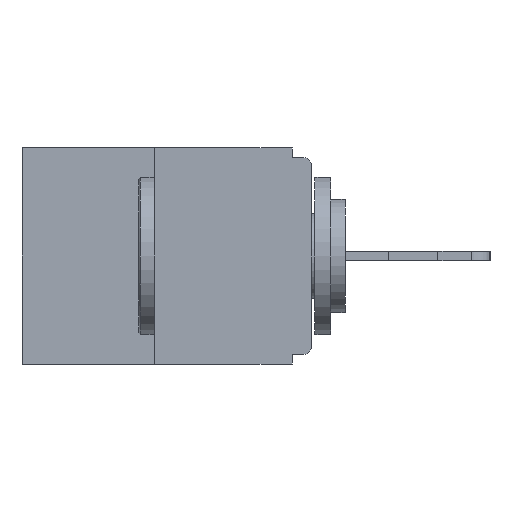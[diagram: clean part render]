
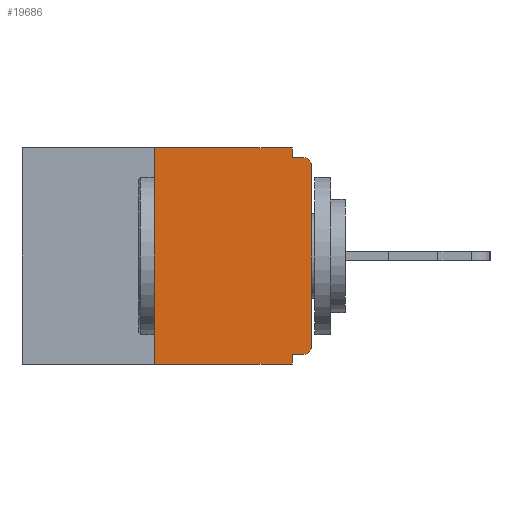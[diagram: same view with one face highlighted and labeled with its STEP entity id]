
A CAD part, left-side view. The second image highlights one B-rep face of the part: STEP entity #19686.
In plain terms, the highlighted planar face has unit normal (-1, 0, 0).
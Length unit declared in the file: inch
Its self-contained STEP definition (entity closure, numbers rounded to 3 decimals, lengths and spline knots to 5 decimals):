
#166 = EDGE_CURVE ( 'NONE', #26643, #11274, #13136, .T. ) ;
#440 = AXIS2_PLACEMENT_3D ( 'NONE', #13246, #17662, #4589 ) ;
#574 = VERTEX_POINT ( 'NONE', #23332 ) ;
#845 = VECTOR ( 'NONE', #21082, 39.37008 ) ;
#1140 = ORIENTED_EDGE ( 'NONE', *, *, #15263, .F. ) ;
#2110 = DIRECTION ( 'NONE',  ( 0., 0., 1. ) ) ;
#2304 = CARTESIAN_POINT ( 'NONE',  ( 0., 0.015, -0.328 ) ) ;
#2438 = AXIS2_PLACEMENT_3D ( 'NONE', #19368, #6268, #21599 ) ;
#2538 = EDGE_CURVE ( 'NONE', #574, #8036, #25478, .T. ) ;
#3503 = LINE ( 'NONE', #9807, #14394 ) ;
#3701 = EDGE_CURVE ( 'NONE', #25444, #11274, #28105, .T. ) ;
#4238 = CARTESIAN_POINT ( 'NONE',  ( 0., 0.25, 0. ) ) ;
#4418 = LINE ( 'NONE', #28301, #27008 ) ;
#4589 = DIRECTION ( 'NONE',  ( 0., 0., -1. ) ) ;
#4833 = CARTESIAN_POINT ( 'NONE',  ( 0., 0., -0.313 ) ) ;
#4880 = EDGE_CURVE ( 'NONE', #6630, #25444, #8194, .T. ) ;
#5594 = CARTESIAN_POINT ( 'NONE',  ( 0., 0.46, 0. ) ) ;
#5620 = ORIENTED_EDGE ( 'NONE', *, *, #4880, .F. ) ;
#5978 = VECTOR ( 'NONE', #16418, 39.37008 ) ;
#6268 = DIRECTION ( 'NONE',  ( -1., 0., 0. ) ) ;
#6456 = DIRECTION ( 'NONE',  ( -1., 0., 0. ) ) ;
#6630 = VERTEX_POINT ( 'NONE', #2304 ) ;
#6703 = PLANE ( 'NONE',  #440 ) ;
#7057 = CARTESIAN_POINT ( 'NONE',  ( 0., 0., -0.328 ) ) ;
#7600 = CARTESIAN_POINT ( 'NONE',  ( 0., 0.015, -0.015 ) ) ;
#7668 = ORIENTED_EDGE ( 'NONE', *, *, #166, .T. ) ;
#7722 = EDGE_CURVE ( 'NONE', #6630, #25954, #27837, .T. ) ;
#8036 = VERTEX_POINT ( 'NONE', #7600 ) ;
#8194 = LINE ( 'NONE', #7057, #19138 ) ;
#9807 = CARTESIAN_POINT ( 'NONE',  ( 0., 0.031, 0. ) ) ;
#10036 = CARTESIAN_POINT ( 'NONE',  ( 0., 0.25, 0. ) ) ;
#10815 = EDGE_LOOP ( 'NONE', ( #11398, #1140, #7668, #15805, #5620, #17919, #14132, #14807, #22090, #17585 ) ) ;
#11274 = VERTEX_POINT ( 'NONE', #26766 ) ;
#11317 = CARTESIAN_POINT ( 'NONE',  ( 0., 0.031, 0. ) ) ;
#11398 = ORIENTED_EDGE ( 'NONE', *, *, #13222, .F. ) ;
#11785 = LINE ( 'NONE', #5594, #5978 ) ;
#12475 = VECTOR ( 'NONE', #22226, 39.37008 ) ;
#13136 = LINE ( 'NONE', #22849, #12475 ) ;
#13222 = EDGE_CURVE ( 'NONE', #26396, #16299, #11785, .T. ) ;
#13244 = DIRECTION ( 'NONE',  ( 0., 0., -1. ) ) ;
#13246 = CARTESIAN_POINT ( 'NONE',  ( 0., 0.46, 0. ) ) ;
#13411 = EDGE_CURVE ( 'NONE', #14710, #8036, #24481, .T. ) ;
#13449 = CARTESIAN_POINT ( 'NONE',  ( 0., 0.031, -0.343 ) ) ;
#14132 = ORIENTED_EDGE ( 'NONE', *, *, #19606, .T. ) ;
#14394 = VECTOR ( 'NONE', #18508, 39.37008 ) ;
#14710 = VERTEX_POINT ( 'NONE', #19495 ) ;
#14807 = ORIENTED_EDGE ( 'NONE', *, *, #13411, .T. ) ;
#15263 = EDGE_CURVE ( 'NONE', #26643, #26396, #18295, .T. ) ;
#15805 = ORIENTED_EDGE ( 'NONE', *, *, #3701, .F. ) ;
#16299 = VERTEX_POINT ( 'NONE', #11317 ) ;
#16390 = VECTOR ( 'NONE', #13244, 39.37008 ) ;
#16418 = DIRECTION ( 'NONE',  ( 0., -1., 0. ) ) ;
#17585 = ORIENTED_EDGE ( 'NONE', *, *, #20485, .F. ) ;
#17662 = DIRECTION ( 'NONE',  ( 1., 0., 0. ) ) ;
#17919 = ORIENTED_EDGE ( 'NONE', *, *, #7722, .T. ) ;
#18295 = LINE ( 'NONE', #10036, #845 ) ;
#18508 = DIRECTION ( 'NONE',  ( 0., 0., -1. ) ) ;
#18963 = DIRECTION ( 'NONE',  ( 0., 1., 0. ) ) ;
#19112 = FACE_OUTER_BOUND ( 'NONE', #10815, .T. ) ;
#19138 = VECTOR ( 'NONE', #18963, 39.37008 ) ;
#19368 = CARTESIAN_POINT ( 'NONE',  ( 0., 0.015, -0.03 ) ) ;
#19495 = CARTESIAN_POINT ( 'NONE',  ( 0., 0., -0.03 ) ) ;
#19562 = CARTESIAN_POINT ( 'NONE',  ( 0., 0.015, -0.313 ) ) ;
#19606 = EDGE_CURVE ( 'NONE', #25954, #14710, #4418, .T. ) ;
#19686 = ADVANCED_FACE ( 'NONE', ( #19112 ), #6703, .F. ) ;
#20485 = EDGE_CURVE ( 'NONE', #16299, #574, #3503, .T. ) ;
#21082 = DIRECTION ( 'NONE',  ( 0., 0., 1. ) ) ;
#21599 = DIRECTION ( 'NONE',  ( 0., 0., -1. ) ) ;
#21788 = DIRECTION ( 'NONE',  ( 0., 0., -1. ) ) ;
#22090 = ORIENTED_EDGE ( 'NONE', *, *, #2538, .F. ) ;
#22226 = DIRECTION ( 'NONE',  ( 0., -1., 0. ) ) ;
#22294 = CARTESIAN_POINT ( 'NONE',  ( 0., 0.031, -0.328 ) ) ;
#22849 = CARTESIAN_POINT ( 'NONE',  ( 0., 0.46, -0.343 ) ) ;
#23332 = CARTESIAN_POINT ( 'NONE',  ( 0., 0.031, -0.015 ) ) ;
#24481 = CIRCLE ( 'NONE', #2438, 0.015 ) ;
#24502 = DIRECTION ( 'NONE',  ( 0., -1., 0. ) ) ;
#24795 = VECTOR ( 'NONE', #24502, 39.37008 ) ;
#25444 = VERTEX_POINT ( 'NONE', #22294 ) ;
#25478 = LINE ( 'NONE', #26640, #24795 ) ;
#25661 = CARTESIAN_POINT ( 'NONE',  ( 0., 0.25, -0.343 ) ) ;
#25954 = VERTEX_POINT ( 'NONE', #4833 ) ;
#26396 = VERTEX_POINT ( 'NONE', #4238 ) ;
#26640 = CARTESIAN_POINT ( 'NONE',  ( 0., 0., -0.015 ) ) ;
#26643 = VERTEX_POINT ( 'NONE', #25661 ) ;
#26766 = CARTESIAN_POINT ( 'NONE',  ( 0., 0.031, -0.343 ) ) ;
#27008 = VECTOR ( 'NONE', #2110, 39.37008 ) ;
#27076 = AXIS2_PLACEMENT_3D ( 'NONE', #19562, #6456, #21788 ) ;
#27837 = CIRCLE ( 'NONE', #27076, 0.015 ) ;
#28105 = LINE ( 'NONE', #13449, #16390 ) ;
#28301 = CARTESIAN_POINT ( 'NONE',  ( 0., 0., 0. ) ) ;
